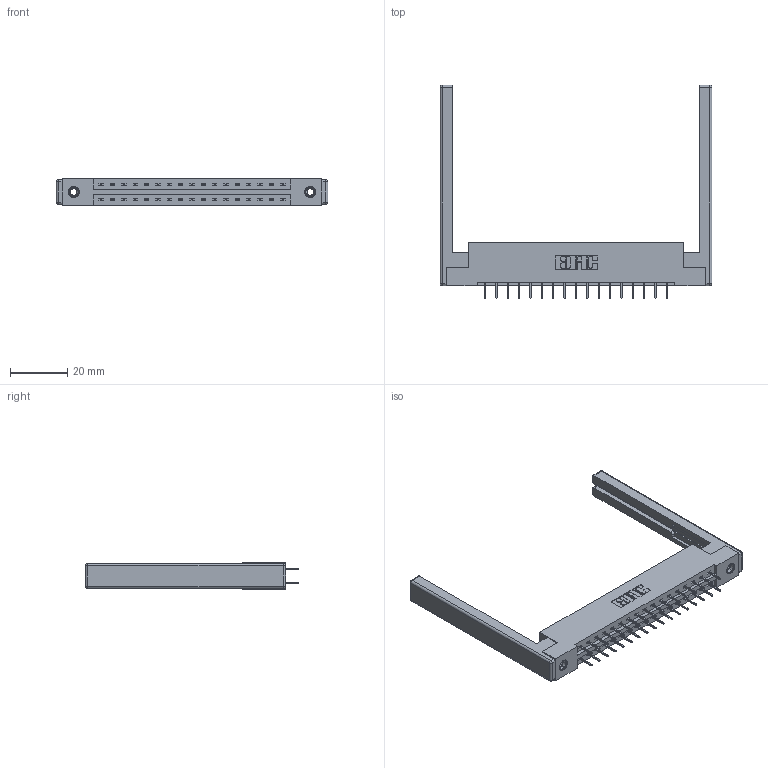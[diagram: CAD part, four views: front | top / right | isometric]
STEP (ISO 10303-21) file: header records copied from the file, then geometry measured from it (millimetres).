
FILE_DESCRIPTION (( 'STEP AP203' ), '1' );
FILE_NAME ('337-034-524-268.STEP', '2019-10-08T20:02:44', ( '' ), ( '' ), 'SwSTEP 2.0', 'SolidWorks 2016', '' );
FILE_SCHEMA (( 'CONFIG_CONTROL_DESIGN' ));
Length unit declared in the file: inch
Products named in the file (5): 337 Part_Flush Mounting Lugs - 0.156 Dia-TI; 345-250-001_345-250-001-102; 307-220-068; 337-034-524-268; 345-292-001_345-293-124
Assembly tree (39 placements, depth 2):
  337-034-524-268
    337 Part_Flush Mounting Lugs - 0.156 Dia-TI
    345-292-001_345-293-124  x34
    345-250-001_345-250-001-102  x2
    307-220-068  x2
Bounding box: 94.79 x 74.43 x 9.4 mm (x, y, z)
Volume: 13990.6 mm3; surface area: 14491.5 mm2
Topology: 39 solids, 39 shells, 2240 faces, 6311 edges, 4050 vertices
Faces by surface type: plane 1654, cylinder 562, cone 12, sphere 8, torus 4
Entity records: 19248 total; most frequent: CARTESIAN_POINT 3227, ORIENTED_EDGE 3152, DIRECTION 2862, EDGE_CURVE 1576, LINE 1402, VECTOR 1402, VERTEX_POINT 1038, AXIS2_PLACEMENT_3D 730
